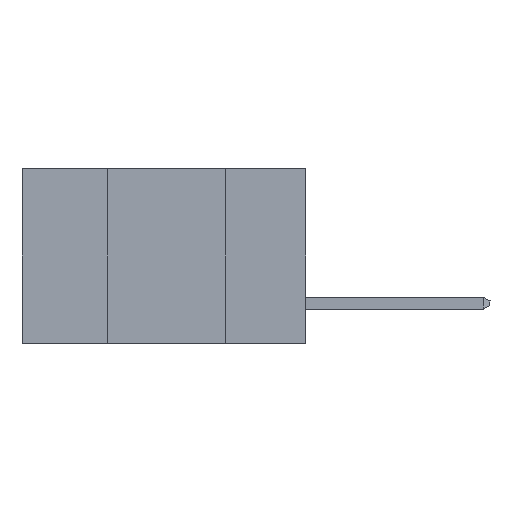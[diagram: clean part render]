
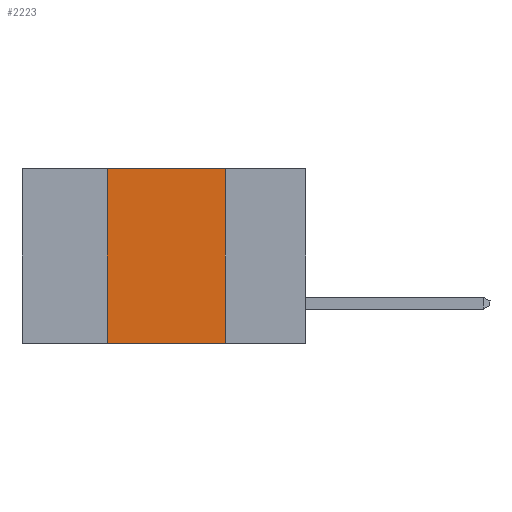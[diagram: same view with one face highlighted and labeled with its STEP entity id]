
A CAD part, left-side view. The second image highlights one B-rep face of the part: STEP entity #2223.
In plain terms, the highlighted planar face has unit normal (-1, 0, 0).
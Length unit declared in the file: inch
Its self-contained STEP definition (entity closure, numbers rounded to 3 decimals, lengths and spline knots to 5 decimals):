
#59 = FACE_OUTER_BOUND ( 'NONE', #15989, .T. ) ;
#887 = EDGE_CURVE ( 'NONE', #15412, #12094, #18711, .T. ) ;
#938 = DIRECTION ( 'NONE',  ( 0., 0., 1. ) ) ;
#1302 = LINE ( 'NONE', #8810, #17283 ) ;
#2223 = ADVANCED_FACE ( 'NONE', ( #59 ), #18434, .F. ) ;
#2236 = AXIS2_PLACEMENT_3D ( 'NONE', #15175, #15248, #6033 ) ;
#2499 = CARTESIAN_POINT ( 'NONE',  ( 0., 0.42, 0. ) ) ;
#2615 = DIRECTION ( 'NONE',  ( 0., -1., 0. ) ) ;
#2868 = ORIENTED_EDGE ( 'NONE', *, *, #887, .F. ) ;
#4464 = ORIENTED_EDGE ( 'NONE', *, *, #13080, .F. ) ;
#4963 = LINE ( 'NONE', #10874, #14983 ) ;
#6033 = DIRECTION ( 'NONE',  ( 0., 0., -1. ) ) ;
#6954 = VECTOR ( 'NONE', #7358, 39.37008 ) ;
#7358 = DIRECTION ( 'NONE',  ( 0., 0., -1. ) ) ;
#7800 = VERTEX_POINT ( 'NONE', #16997 ) ;
#8810 = CARTESIAN_POINT ( 'NONE',  ( 0., 0.6, -0.37 ) ) ;
#9631 = LINE ( 'NONE', #18040, #6954 ) ;
#10874 = CARTESIAN_POINT ( 'NONE',  ( 0., 0.6, 0. ) ) ;
#12094 = VERTEX_POINT ( 'NONE', #16549 ) ;
#12383 = DIRECTION ( 'NONE',  ( 0., -1., 0. ) ) ;
#13080 = EDGE_CURVE ( 'NONE', #12094, #7800, #4963, .T. ) ;
#14983 = VECTOR ( 'NONE', #12383, 39.37008 ) ;
#15175 = CARTESIAN_POINT ( 'NONE',  ( 0., 0.6, 0. ) ) ;
#15248 = DIRECTION ( 'NONE',  ( 1., 0., 0. ) ) ;
#15412 = VERTEX_POINT ( 'NONE', #16491 ) ;
#15989 = EDGE_LOOP ( 'NONE', ( #19081, #4464, #2868, #17213 ) ) ;
#16258 = EDGE_CURVE ( 'NONE', #15412, #17714, #1302, .T. ) ;
#16307 = VECTOR ( 'NONE', #938, 39.37008 ) ;
#16491 = CARTESIAN_POINT ( 'NONE',  ( 0., 0.42, -0.37 ) ) ;
#16549 = CARTESIAN_POINT ( 'NONE',  ( 0., 0.42, 0. ) ) ;
#16997 = CARTESIAN_POINT ( 'NONE',  ( 0., 0.17, 0. ) ) ;
#17213 = ORIENTED_EDGE ( 'NONE', *, *, #16258, .T. ) ;
#17283 = VECTOR ( 'NONE', #2615, 39.37008 ) ;
#17714 = VERTEX_POINT ( 'NONE', #17726 ) ;
#17726 = CARTESIAN_POINT ( 'NONE',  ( 0., 0.17, -0.37 ) ) ;
#17784 = EDGE_CURVE ( 'NONE', #7800, #17714, #9631, .T. ) ;
#18040 = CARTESIAN_POINT ( 'NONE',  ( 0., 0.17, 0. ) ) ;
#18434 = PLANE ( 'NONE',  #2236 ) ;
#18711 = LINE ( 'NONE', #2499, #16307 ) ;
#19081 = ORIENTED_EDGE ( 'NONE', *, *, #17784, .F. ) ;
